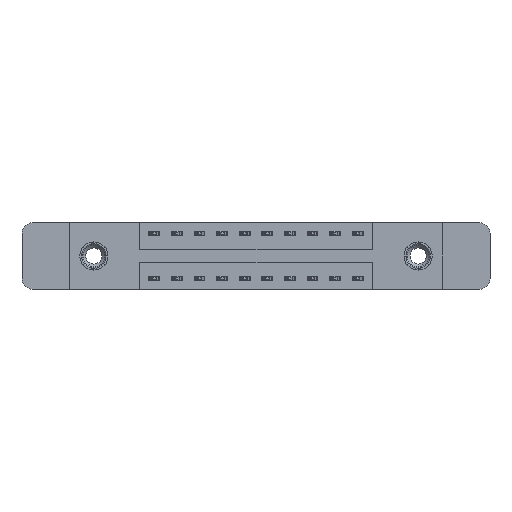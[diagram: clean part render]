
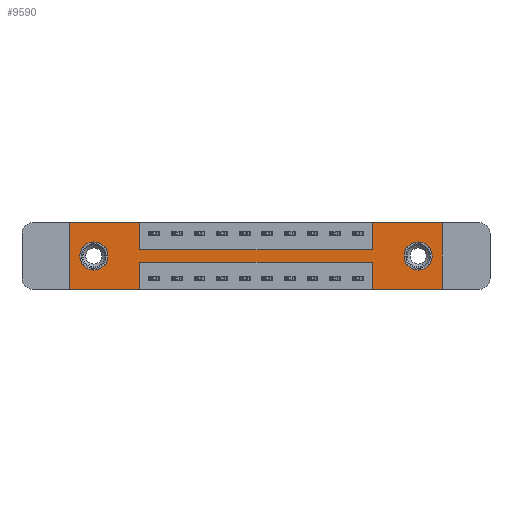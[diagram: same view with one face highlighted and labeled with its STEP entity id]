
A CAD part, front view. The second image highlights one B-rep face of the part: STEP entity #9590.
In plain terms, the highlighted planar face has unit normal (0, -1, 0).
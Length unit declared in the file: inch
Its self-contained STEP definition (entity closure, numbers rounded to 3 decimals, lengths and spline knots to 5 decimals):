
#28 = VERTEX_POINT ( 'NONE', #12284 ) ;
#503 = VERTEX_POINT ( 'NONE', #4922 ) ;
#722 = ORIENTED_EDGE ( 'NONE', *, *, #1851, .F. ) ;
#812 = CARTESIAN_POINT ( 'NONE',  ( 0., 0., -0.37 ) ) ;
#821 = CARTESIAN_POINT ( 'NONE',  ( 0.1325, 0., -0.185 ) ) ;
#838 = VECTOR ( 'NONE', #11810, 39.37008 ) ;
#848 = DIRECTION ( 'NONE',  ( 1., 0., 0. ) ) ;
#1005 = CARTESIAN_POINT ( 'NONE',  ( 0.1325, 0., -0.263 ) ) ;
#1124 = VECTOR ( 'NONE', #848, 39.37008 ) ;
#1192 = ORIENTED_EDGE ( 'NONE', *, *, #7389, .F. ) ;
#1322 = CARTESIAN_POINT ( 'NONE',  ( 0.3875, 0., -0.15 ) ) ;
#1387 = CARTESIAN_POINT ( 'NONE',  ( 0.3875, 0., -0.22 ) ) ;
#1389 = VECTOR ( 'NONE', #12009, 39.37008 ) ;
#1501 = CARTESIAN_POINT ( 'NONE',  ( 0., 0., -0.37 ) ) ;
#1601 = EDGE_CURVE ( 'NONE', #14191, #15095, #11658, .T. ) ;
#1758 = ORIENTED_EDGE ( 'NONE', *, *, #2091, .T. ) ;
#1775 = CARTESIAN_POINT ( 'NONE',  ( 1.9275, 0., -0.263 ) ) ;
#1825 = LINE ( 'NONE', #1501, #838 ) ;
#1834 = CARTESIAN_POINT ( 'NONE',  ( 0.3875, 0., -0.22 ) ) ;
#1851 = EDGE_CURVE ( 'NONE', #11321, #3768, #5004, .T. ) ;
#1919 = CARTESIAN_POINT ( 'NONE',  ( 1.9275, 0., -0.185 ) ) ;
#2091 = EDGE_CURVE ( 'NONE', #7665, #5481, #15462, .T. ) ;
#2133 = ORIENTED_EDGE ( 'NONE', *, *, #1601, .F. ) ;
#2292 = EDGE_CURVE ( 'NONE', #10459, #11321, #12816, .T. ) ;
#2498 = CARTESIAN_POINT ( 'NONE',  ( 0., 0., 0. ) ) ;
#2678 = CARTESIAN_POINT ( 'NONE',  ( 2.06, 0., 0. ) ) ;
#2730 = VECTOR ( 'NONE', #6770, 39.37008 ) ;
#2888 = ORIENTED_EDGE ( 'NONE', *, *, #8655, .T. ) ;
#2932 = VERTEX_POINT ( 'NONE', #14603 ) ;
#3114 = CARTESIAN_POINT ( 'NONE',  ( 0., 0., 0. ) ) ;
#3254 = DIRECTION ( 'NONE',  ( 0., 1., 0. ) ) ;
#3342 = CARTESIAN_POINT ( 'NONE',  ( 1.9275, 0., -0.107 ) ) ;
#3344 = DIRECTION ( 'NONE',  ( 0., 0., 1. ) ) ;
#3415 = DIRECTION ( 'NONE',  ( 0., 1., 0. ) ) ;
#3429 = VERTEX_POINT ( 'NONE', #1775 ) ;
#3449 = ORIENTED_EDGE ( 'NONE', *, *, #9736, .T. ) ;
#3462 = EDGE_CURVE ( 'NONE', #5481, #7665, #6761, .T. ) ;
#3488 = VECTOR ( 'NONE', #15382, 39.37008 ) ;
#3624 = ORIENTED_EDGE ( 'NONE', *, *, #15380, .F. ) ;
#3767 = CIRCLE ( 'NONE', #12015, 0.078 ) ;
#3768 = VERTEX_POINT ( 'NONE', #10724 ) ;
#3841 = AXIS2_PLACEMENT_3D ( 'NONE', #12233, #14438, #14904 ) ;
#4009 = VECTOR ( 'NONE', #13960, 39.37008 ) ;
#4014 = ORIENTED_EDGE ( 'NONE', *, *, #2292, .F. ) ;
#4177 = DIRECTION ( 'NONE',  ( 0., 0., -1. ) ) ;
#4225 = ORIENTED_EDGE ( 'NONE', *, *, #9260, .F. ) ;
#4260 = EDGE_LOOP ( 'NONE', ( #2133, #4876, #1192, #6095, #722, #4014, #15739, #15933, #10729, #4225, #3624, #15916 ) ) ;
#4333 = FACE_OUTER_BOUND ( 'NONE', #4260, .T. ) ;
#4482 = CARTESIAN_POINT ( 'NONE',  ( 1.9275, 0., -0.185 ) ) ;
#4876 = ORIENTED_EDGE ( 'NONE', *, *, #7453, .F. ) ;
#4921 = CARTESIAN_POINT ( 'NONE',  ( 0., 0., -0.37 ) ) ;
#4922 = CARTESIAN_POINT ( 'NONE',  ( 0., 0., 0. ) ) ;
#5004 = LINE ( 'NONE', #2678, #13330 ) ;
#5068 = AXIS2_PLACEMENT_3D ( 'NONE', #821, #10989, #3344 ) ;
#5457 = EDGE_CURVE ( 'NONE', #3768, #11803, #13742, .T. ) ;
#5481 = VERTEX_POINT ( 'NONE', #1005 ) ;
#5796 = EDGE_LOOP ( 'NONE', ( #2888, #3449 ) ) ;
#5918 = AXIS2_PLACEMENT_3D ( 'NONE', #6571, #10643, #4177 ) ;
#6095 = ORIENTED_EDGE ( 'NONE', *, *, #5457, .F. ) ;
#6510 = DIRECTION ( 'NONE',  ( 0., 0., -1. ) ) ;
#6532 = CARTESIAN_POINT ( 'NONE',  ( 1.6725, 0., 0. ) ) ;
#6571 = CARTESIAN_POINT ( 'NONE',  ( 0., 0., -0.37 ) ) ;
#6604 = CARTESIAN_POINT ( 'NONE',  ( 0., 0., 0. ) ) ;
#6633 = CARTESIAN_POINT ( 'NONE',  ( 2.06, 0., 0. ) ) ;
#6761 = CIRCLE ( 'NONE', #3841, 0.078 ) ;
#6770 = DIRECTION ( 'NONE',  ( 0., 0., -1. ) ) ;
#7042 = VERTEX_POINT ( 'NONE', #10173 ) ;
#7295 = CARTESIAN_POINT ( 'NONE',  ( 0.1325, 0., -0.107 ) ) ;
#7389 = EDGE_CURVE ( 'NONE', #11803, #7042, #7636, .T. ) ;
#7453 = EDGE_CURVE ( 'NONE', #7042, #14191, #12794, .T. ) ;
#7636 = LINE ( 'NONE', #13024, #4009 ) ;
#7665 = VERTEX_POINT ( 'NONE', #7295 ) ;
#7946 = LINE ( 'NONE', #6604, #14676 ) ;
#7993 = FACE_BOUND ( 'NONE', #5796, .T. ) ;
#8017 = CARTESIAN_POINT ( 'NONE',  ( 0.3875, 0., 0. ) ) ;
#8096 = EDGE_LOOP ( 'NONE', ( #1758, #8970 ) ) ;
#8513 = EDGE_CURVE ( 'NONE', #15095, #9862, #1825, .T. ) ;
#8655 = EDGE_CURVE ( 'NONE', #16385, #3429, #3767, .T. ) ;
#8805 = AXIS2_PLACEMENT_3D ( 'NONE', #1919, #3415, #11139 ) ;
#8970 = ORIENTED_EDGE ( 'NONE', *, *, #3462, .T. ) ;
#9127 = CARTESIAN_POINT ( 'NONE',  ( 1.6725, 0., -0.37 ) ) ;
#9144 = VERTEX_POINT ( 'NONE', #15120 ) ;
#9260 = EDGE_CURVE ( 'NONE', #503, #28, #7946, .T. ) ;
#9590 = ADVANCED_FACE ( 'NONE', ( #7993, #14316, #4333 ), #15824, .T. ) ;
#9736 = EDGE_CURVE ( 'NONE', #3429, #16385, #10920, .T. ) ;
#9862 = VERTEX_POINT ( 'NONE', #812 ) ;
#9870 = LINE ( 'NONE', #12623, #14674 ) ;
#10080 = DIRECTION ( 'NONE',  ( 0., 0., -1. ) ) ;
#10173 = CARTESIAN_POINT ( 'NONE',  ( 1.6725, 0., -0.22 ) ) ;
#10429 = CARTESIAN_POINT ( 'NONE',  ( 0.3875, 0., -0.37 ) ) ;
#10444 = DIRECTION ( 'NONE',  ( 1., 0., 0. ) ) ;
#10459 = VERTEX_POINT ( 'NONE', #6532 ) ;
#10643 = DIRECTION ( 'NONE',  ( 0., -1., 0. ) ) ;
#10724 = CARTESIAN_POINT ( 'NONE',  ( 2.06, 0., -0.37 ) ) ;
#10729 = ORIENTED_EDGE ( 'NONE', *, *, #10832, .F. ) ;
#10832 = EDGE_CURVE ( 'NONE', #28, #9144, #14091, .T. ) ;
#10833 = VECTOR ( 'NONE', #6510, 39.37008 ) ;
#10920 = CIRCLE ( 'NONE', #8805, 0.078 ) ;
#10989 = DIRECTION ( 'NONE',  ( 0., 1., 0. ) ) ;
#11139 = DIRECTION ( 'NONE',  ( 0., 0., -1. ) ) ;
#11321 = VERTEX_POINT ( 'NONE', #6633 ) ;
#11658 = LINE ( 'NONE', #10429, #2730 ) ;
#11803 = VERTEX_POINT ( 'NONE', #9127 ) ;
#11810 = DIRECTION ( 'NONE',  ( -1., 0., 0. ) ) ;
#12009 = DIRECTION ( 'NONE',  ( 0., 0., 1. ) ) ;
#12015 = AXIS2_PLACEMENT_3D ( 'NONE', #4482, #3254, #13642 ) ;
#12233 = CARTESIAN_POINT ( 'NONE',  ( 0.1325, 0., -0.185 ) ) ;
#12284 = CARTESIAN_POINT ( 'NONE',  ( 0.3875, 0., 0. ) ) ;
#12332 = DIRECTION ( 'NONE',  ( -1., 0., 0. ) ) ;
#12568 = DIRECTION ( 'NONE',  ( 1., 0., 0. ) ) ;
#12623 = CARTESIAN_POINT ( 'NONE',  ( 1.6725, 0., 0. ) ) ;
#12794 = LINE ( 'NONE', #1387, #3488 ) ;
#12816 = LINE ( 'NONE', #2498, #13588 ) ;
#13024 = CARTESIAN_POINT ( 'NONE',  ( 1.6725, 0., -0.37 ) ) ;
#13330 = VECTOR ( 'NONE', #10080, 39.37008 ) ;
#13529 = VECTOR ( 'NONE', #12332, 39.37008 ) ;
#13588 = VECTOR ( 'NONE', #12568, 39.37008 ) ;
#13642 = DIRECTION ( 'NONE',  ( 0., 0., -1. ) ) ;
#13656 = EDGE_CURVE ( 'NONE', #2932, #10459, #9870, .T. ) ;
#13742 = LINE ( 'NONE', #4921, #13529 ) ;
#13960 = DIRECTION ( 'NONE',  ( 0., 0., 1. ) ) ;
#14091 = LINE ( 'NONE', #8017, #10833 ) ;
#14191 = VERTEX_POINT ( 'NONE', #1834 ) ;
#14316 = FACE_BOUND ( 'NONE', #8096, .T. ) ;
#14438 = DIRECTION ( 'NONE',  ( 0., 1., 0. ) ) ;
#14603 = CARTESIAN_POINT ( 'NONE',  ( 1.6725, 0., -0.15 ) ) ;
#14672 = LINE ( 'NONE', #3114, #1389 ) ;
#14674 = VECTOR ( 'NONE', #14965, 39.37008 ) ;
#14676 = VECTOR ( 'NONE', #10444, 39.37008 ) ;
#14904 = DIRECTION ( 'NONE',  ( 0., 0., 1. ) ) ;
#14965 = DIRECTION ( 'NONE',  ( 0., 0., 1. ) ) ;
#15095 = VERTEX_POINT ( 'NONE', #16115 ) ;
#15120 = CARTESIAN_POINT ( 'NONE',  ( 0.3875, 0., -0.15 ) ) ;
#15380 = EDGE_CURVE ( 'NONE', #9862, #503, #14672, .T. ) ;
#15382 = DIRECTION ( 'NONE',  ( -1., 0., 0. ) ) ;
#15462 = CIRCLE ( 'NONE', #5068, 0.078 ) ;
#15594 = EDGE_CURVE ( 'NONE', #9144, #2932, #16098, .T. ) ;
#15739 = ORIENTED_EDGE ( 'NONE', *, *, #13656, .F. ) ;
#15824 = PLANE ( 'NONE',  #5918 ) ;
#15916 = ORIENTED_EDGE ( 'NONE', *, *, #8513, .F. ) ;
#15933 = ORIENTED_EDGE ( 'NONE', *, *, #15594, .F. ) ;
#16098 = LINE ( 'NONE', #1322, #1124 ) ;
#16115 = CARTESIAN_POINT ( 'NONE',  ( 0.3875, 0., -0.37 ) ) ;
#16385 = VERTEX_POINT ( 'NONE', #3342 ) ;
